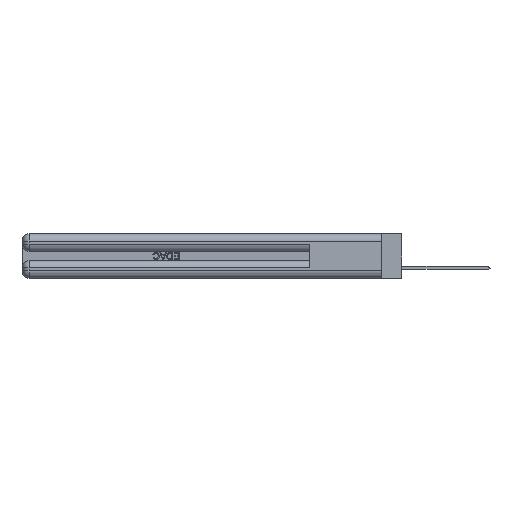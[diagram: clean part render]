
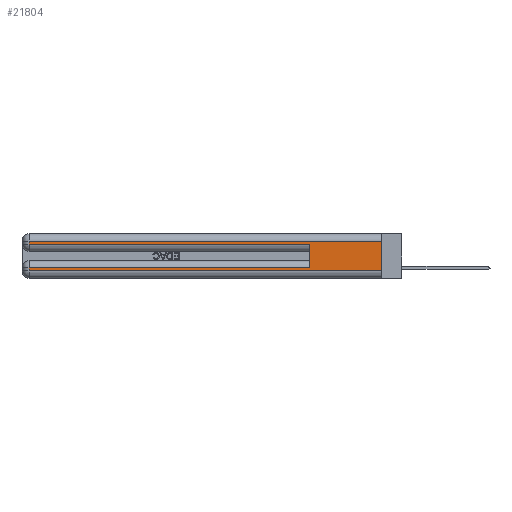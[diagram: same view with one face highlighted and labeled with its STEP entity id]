
A CAD part, left-side view. The second image highlights one B-rep face of the part: STEP entity #21804.
In plain terms, the highlighted planar face has unit normal (-1, 0, 0).
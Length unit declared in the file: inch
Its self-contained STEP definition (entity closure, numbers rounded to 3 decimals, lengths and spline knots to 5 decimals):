
#320 = VERTEX_POINT ( 'NONE', #45751 ) ;
#515 = PLANE ( 'NONE',  #8052 ) ;
#1745 = EDGE_CURVE ( 'NONE', #27446, #320, #7825, .T. ) ;
#2215 = ORIENTED_EDGE ( 'NONE', *, *, #21742, .F. ) ;
#2738 = ORIENTED_EDGE ( 'NONE', *, *, #21653, .T. ) ;
#3109 = DIRECTION ( 'NONE',  ( 0., 0., 1. ) ) ;
#3581 = DIRECTION ( 'NONE',  ( 0., 0., -1. ) ) ;
#5173 = DIRECTION ( 'NONE',  ( 1., 0., 0. ) ) ;
#6346 = DIRECTION ( 'NONE',  ( 0., 0., -1. ) ) ;
#7366 = DIRECTION ( 'NONE',  ( 0., 1., 0. ) ) ;
#7668 = EDGE_CURVE ( 'NONE', #39695, #320, #39306, .T. ) ;
#7825 = LINE ( 'NONE', #29740, #9691 ) ;
#8052 = AXIS2_PLACEMENT_3D ( 'NONE', #49288, #5173, #21487 ) ;
#9247 = LINE ( 'NONE', #9499, #36219 ) ;
#9499 = CARTESIAN_POINT ( 'NONE',  ( 0., 0., 0.31 ) ) ;
#9691 = VECTOR ( 'NONE', #17806, 39.37008 ) ;
#10506 = FACE_OUTER_BOUND ( 'NONE', #48916, .T. ) ;
#13037 = CARTESIAN_POINT ( 'NONE',  ( 0., 0.6, 0.085 ) ) ;
#14494 = CARTESIAN_POINT ( 'NONE',  ( 0., 0., 0.31 ) ) ;
#14740 = VECTOR ( 'NONE', #50706, 39.37008 ) ;
#14770 = ORIENTED_EDGE ( 'NONE', *, *, #1745, .T. ) ;
#15857 = VECTOR ( 'NONE', #7366, 39.37008 ) ;
#16074 = VECTOR ( 'NONE', #6346, 39.37008 ) ;
#16402 = ORIENTED_EDGE ( 'NONE', *, *, #17904, .T. ) ;
#17806 = DIRECTION ( 'NONE',  ( 0., -1., 0. ) ) ;
#17904 = EDGE_CURVE ( 'NONE', #45773, #51176, #27856, .T. ) ;
#18082 = CARTESIAN_POINT ( 'NONE',  ( 0., 2.94, 0.31 ) ) ;
#19856 = ORIENTED_EDGE ( 'NONE', *, *, #7668, .F. ) ;
#20285 = EDGE_CURVE ( 'NONE', #46860, #45773, #46953, .T. ) ;
#21487 = DIRECTION ( 'NONE',  ( 0., 0., -1. ) ) ;
#21653 = EDGE_CURVE ( 'NONE', #39695, #46860, #9247, .T. ) ;
#21742 = EDGE_CURVE ( 'NONE', #31172, #51176, #26144, .T. ) ;
#21804 = ADVANCED_FACE ( 'NONE', ( #10506 ), #515, .F. ) ;
#21985 = ORIENTED_EDGE ( 'NONE', *, *, #20285, .T. ) ;
#22801 = CARTESIAN_POINT ( 'NONE',  ( 0., 0., 0.37 ) ) ;
#23970 = CARTESIAN_POINT ( 'NONE',  ( 0., 0.6, 0.145 ) ) ;
#25089 = ORIENTED_EDGE ( 'NONE', *, *, #45851, .T. ) ;
#25143 = CARTESIAN_POINT ( 'NONE',  ( 0., 2.94, 0.37 ) ) ;
#26144 = LINE ( 'NONE', #23970, #28068 ) ;
#26442 = CARTESIAN_POINT ( 'NONE',  ( 0., 2.94, 0.285 ) ) ;
#27446 = VERTEX_POINT ( 'NONE', #45139 ) ;
#27856 = LINE ( 'NONE', #45042, #34779 ) ;
#28068 = VECTOR ( 'NONE', #3109, 39.37008 ) ;
#29740 = CARTESIAN_POINT ( 'NONE',  ( 0., 0., 0.06 ) ) ;
#31172 = VERTEX_POINT ( 'NONE', #13037 ) ;
#34469 = CARTESIAN_POINT ( 'NONE',  ( 0., 0.6, 0.285 ) ) ;
#34779 = VECTOR ( 'NONE', #49761, 39.37008 ) ;
#34877 = EDGE_CURVE ( 'NONE', #31172, #47688, #40275, .T. ) ;
#36219 = VECTOR ( 'NONE', #47213, 39.37008 ) ;
#37074 = CARTESIAN_POINT ( 'NONE',  ( 0., 2.94, 0.085 ) ) ;
#39306 = LINE ( 'NONE', #22801, #16074 ) ;
#39695 = VERTEX_POINT ( 'NONE', #14494 ) ;
#40275 = LINE ( 'NONE', #42702, #15857 ) ;
#41602 = ORIENTED_EDGE ( 'NONE', *, *, #34877, .T. ) ;
#42702 = CARTESIAN_POINT ( 'NONE',  ( 0., 0., 0.085 ) ) ;
#43486 = LINE ( 'NONE', #25143, #14740 ) ;
#45042 = CARTESIAN_POINT ( 'NONE',  ( 0., 0., 0.285 ) ) ;
#45139 = CARTESIAN_POINT ( 'NONE',  ( 0., 2.94, 0.06 ) ) ;
#45751 = CARTESIAN_POINT ( 'NONE',  ( 0., 0., 0.06 ) ) ;
#45773 = VERTEX_POINT ( 'NONE', #26442 ) ;
#45851 = EDGE_CURVE ( 'NONE', #47688, #27446, #43486, .T. ) ;
#46860 = VERTEX_POINT ( 'NONE', #18082 ) ;
#46953 = LINE ( 'NONE', #47936, #49426 ) ;
#47213 = DIRECTION ( 'NONE',  ( 0., 1., 0. ) ) ;
#47688 = VERTEX_POINT ( 'NONE', #37074 ) ;
#47936 = CARTESIAN_POINT ( 'NONE',  ( 0., 2.94, 0.37 ) ) ;
#48916 = EDGE_LOOP ( 'NONE', ( #19856, #2738, #21985, #16402, #2215, #41602, #25089, #14770 ) ) ;
#49288 = CARTESIAN_POINT ( 'NONE',  ( 0., 0., 0.37 ) ) ;
#49426 = VECTOR ( 'NONE', #3581, 39.37008 ) ;
#49761 = DIRECTION ( 'NONE',  ( 0., -1., 0. ) ) ;
#50706 = DIRECTION ( 'NONE',  ( 0., 0., -1. ) ) ;
#51176 = VERTEX_POINT ( 'NONE', #34469 ) ;
